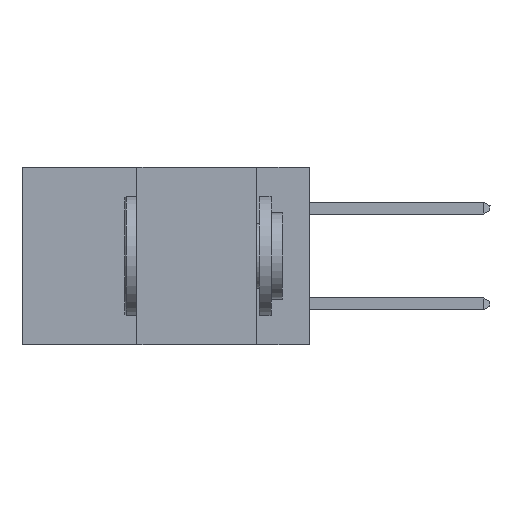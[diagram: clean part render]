
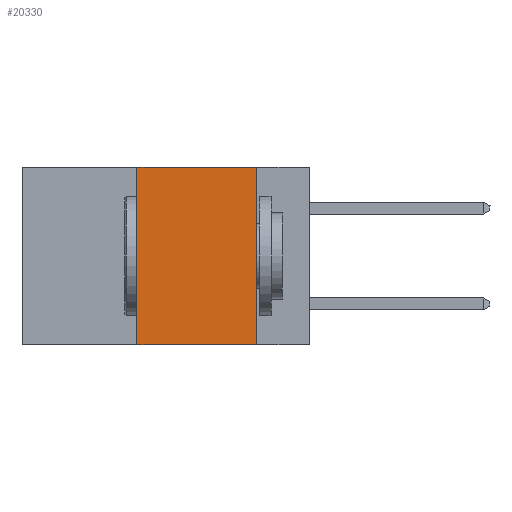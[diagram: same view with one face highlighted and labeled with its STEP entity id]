
A CAD part, left-side view. The second image highlights one B-rep face of the part: STEP entity #20330.
In plain terms, the highlighted planar face has unit normal (-1, 0, 0).
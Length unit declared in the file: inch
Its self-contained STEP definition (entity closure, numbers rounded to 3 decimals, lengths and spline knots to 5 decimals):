
#246 = CARTESIAN_POINT ( 'NONE',  ( 0., 0.6, -0.37 ) ) ;
#791 = CARTESIAN_POINT ( 'NONE',  ( 0., 0.11, 0. ) ) ;
#1859 = CARTESIAN_POINT ( 'NONE',  ( 0., 0.6, 0. ) ) ;
#2660 = ORIENTED_EDGE ( 'NONE', *, *, #15738, .T. ) ;
#2751 = VECTOR ( 'NONE', #25826, 39.37008 ) ;
#3323 = VECTOR ( 'NONE', #14181, 39.37008 ) ;
#4181 = DIRECTION ( 'NONE',  ( 1., 0., 0. ) ) ;
#5685 = ORIENTED_EDGE ( 'NONE', *, *, #28945, .F. ) ;
#6642 = DIRECTION ( 'NONE',  ( 0., -1., 0. ) ) ;
#7411 = FACE_OUTER_BOUND ( 'NONE', #14146, .T. ) ;
#8157 = VERTEX_POINT ( 'NONE', #9347 ) ;
#8703 = EDGE_CURVE ( 'NONE', #8157, #13105, #27618, .T. ) ;
#8933 = EDGE_CURVE ( 'NONE', #22781, #8157, #15059, .T. ) ;
#9347 = CARTESIAN_POINT ( 'NONE',  ( 0., 0.36, 0. ) ) ;
#11477 = ORIENTED_EDGE ( 'NONE', *, *, #8933, .F. ) ;
#11679 = CARTESIAN_POINT ( 'NONE',  ( 0., 0.11, -0.37 ) ) ;
#13105 = VERTEX_POINT ( 'NONE', #791 ) ;
#14146 = EDGE_LOOP ( 'NONE', ( #5685, #23335, #11477, #2660 ) ) ;
#14181 = DIRECTION ( 'NONE',  ( 0., -1., 0. ) ) ;
#15059 = LINE ( 'NONE', #28097, #2751 ) ;
#15446 = VECTOR ( 'NONE', #6642, 39.37008 ) ;
#15665 = LINE ( 'NONE', #246, #3323 ) ;
#15738 = EDGE_CURVE ( 'NONE', #22781, #17358, #15665, .T. ) ;
#16679 = CARTESIAN_POINT ( 'NONE',  ( 0., 0.11, 0. ) ) ;
#16940 = VECTOR ( 'NONE', #18972, 39.37008 ) ;
#17358 = VERTEX_POINT ( 'NONE', #11679 ) ;
#18041 = PLANE ( 'NONE',  #29852 ) ;
#18972 = DIRECTION ( 'NONE',  ( 0., 0., -1. ) ) ;
#19737 = CARTESIAN_POINT ( 'NONE',  ( 0., 0.36, -0.37 ) ) ;
#20330 = ADVANCED_FACE ( 'NONE', ( #7411 ), #18041, .F. ) ;
#20346 = DIRECTION ( 'NONE',  ( 0., 0., -1. ) ) ;
#22781 = VERTEX_POINT ( 'NONE', #19737 ) ;
#23045 = LINE ( 'NONE', #16679, #16940 ) ;
#23335 = ORIENTED_EDGE ( 'NONE', *, *, #8703, .F. ) ;
#25826 = DIRECTION ( 'NONE',  ( 0., 0., 1. ) ) ;
#27215 = CARTESIAN_POINT ( 'NONE',  ( 0., 0.6, 0. ) ) ;
#27618 = LINE ( 'NONE', #27215, #15446 ) ;
#28097 = CARTESIAN_POINT ( 'NONE',  ( 0., 0.36, 0. ) ) ;
#28945 = EDGE_CURVE ( 'NONE', #13105, #17358, #23045, .T. ) ;
#29852 = AXIS2_PLACEMENT_3D ( 'NONE', #1859, #4181, #20346 ) ;
